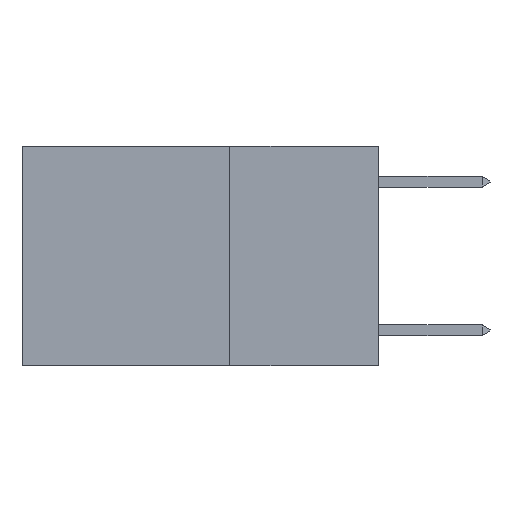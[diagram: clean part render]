
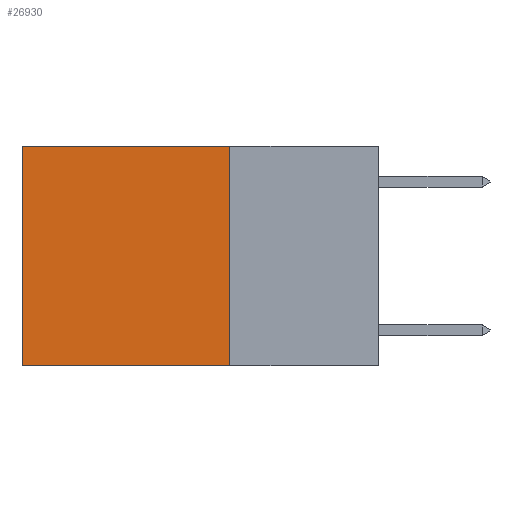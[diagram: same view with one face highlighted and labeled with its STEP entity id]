
A CAD part, left-side view. The second image highlights one B-rep face of the part: STEP entity #26930.
In plain terms, the highlighted planar face has unit normal (-1, 0, 0).
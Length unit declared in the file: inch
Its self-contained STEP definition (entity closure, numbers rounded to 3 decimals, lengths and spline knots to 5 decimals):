
#395 = EDGE_CURVE ( 'NONE', #3638, #25277, #13461, .T. ) ;
#521 = VERTEX_POINT ( 'NONE', #2977 ) ;
#1245 = CARTESIAN_POINT ( 'NONE',  ( 0.2625, 0.25, 0. ) ) ;
#1352 = EDGE_CURVE ( 'NONE', #521, #4677, #10071, .T. ) ;
#1789 = VECTOR ( 'NONE', #2262, 39.37008 ) ;
#2039 = LINE ( 'NONE', #17193, #3331 ) ;
#2262 = DIRECTION ( 'NONE',  ( 0., 0., -1. ) ) ;
#2977 = CARTESIAN_POINT ( 'NONE',  ( 0.2625, 0.25, 0. ) ) ;
#3331 = VECTOR ( 'NONE', #4265, 39.37008 ) ;
#3447 = ORIENTED_EDGE ( 'NONE', *, *, #3735, .T. ) ;
#3638 = VERTEX_POINT ( 'NONE', #10317 ) ;
#3735 = EDGE_CURVE ( 'NONE', #521, #3638, #3983, .T. ) ;
#3983 = LINE ( 'NONE', #26298, #19463 ) ;
#4265 = DIRECTION ( 'NONE',  ( 0., 1., 0. ) ) ;
#4469 = CARTESIAN_POINT ( 'NONE',  ( 0.2625, 0.25, -0.37 ) ) ;
#4677 = VERTEX_POINT ( 'NONE', #4469 ) ;
#7574 = DIRECTION ( 'NONE',  ( 0., 0., -1. ) ) ;
#10071 = LINE ( 'NONE', #1245, #16388 ) ;
#10317 = CARTESIAN_POINT ( 'NONE',  ( 0.2625, 0.6, 0. ) ) ;
#11576 = ORIENTED_EDGE ( 'NONE', *, *, #395, .T. ) ;
#13461 = LINE ( 'NONE', #22385, #1789 ) ;
#13694 = PLANE ( 'NONE',  #15622 ) ;
#14190 = EDGE_CURVE ( 'NONE', #4677, #25277, #2039, .T. ) ;
#15599 = CARTESIAN_POINT ( 'NONE',  ( 0.2625, 0.25, 0. ) ) ;
#15622 = AXIS2_PLACEMENT_3D ( 'NONE', #15599, #15735, #24700 ) ;
#15735 = DIRECTION ( 'NONE',  ( 1., 0., 0. ) ) ;
#16388 = VECTOR ( 'NONE', #7574, 39.37008 ) ;
#16919 = DIRECTION ( 'NONE',  ( 0., 1., 0. ) ) ;
#17014 = ORIENTED_EDGE ( 'NONE', *, *, #1352, .F. ) ;
#17029 = CARTESIAN_POINT ( 'NONE',  ( 0.2625, 0.6, -0.37 ) ) ;
#17193 = CARTESIAN_POINT ( 'NONE',  ( 0.2625, 0.25, -0.37 ) ) ;
#19463 = VECTOR ( 'NONE', #16919, 39.37008 ) ;
#22385 = CARTESIAN_POINT ( 'NONE',  ( 0.2625, 0.6, 0. ) ) ;
#23726 = EDGE_LOOP ( 'NONE', ( #11576, #23898, #17014, #3447 ) ) ;
#23898 = ORIENTED_EDGE ( 'NONE', *, *, #14190, .F. ) ;
#24700 = DIRECTION ( 'NONE',  ( 0., 0., -1. ) ) ;
#25277 = VERTEX_POINT ( 'NONE', #17029 ) ;
#26298 = CARTESIAN_POINT ( 'NONE',  ( 0.2625, 0.25, 0. ) ) ;
#26930 = ADVANCED_FACE ( 'NONE', ( #28969 ), #13694, .F. ) ;
#28969 = FACE_OUTER_BOUND ( 'NONE', #23726, .T. ) ;
